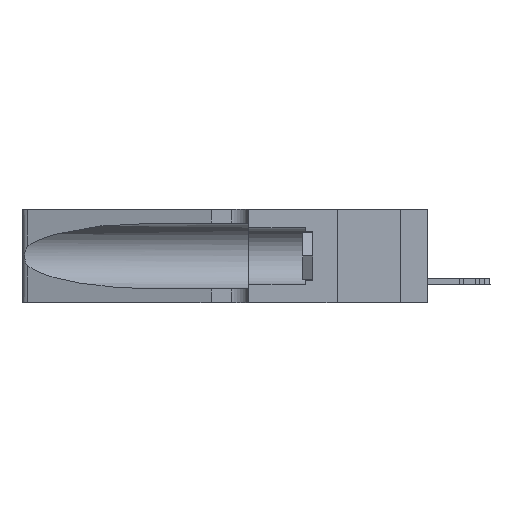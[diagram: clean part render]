
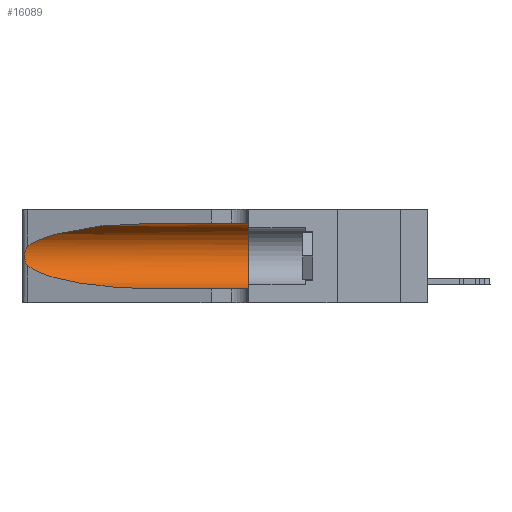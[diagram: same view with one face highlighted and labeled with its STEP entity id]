
A CAD part, left-side view. The second image highlights one B-rep face of the part: STEP entity #16089.
In plain terms, the highlighted cylindrical face has radius 3.308 mm (diameter 6.617 mm), a partial arc.
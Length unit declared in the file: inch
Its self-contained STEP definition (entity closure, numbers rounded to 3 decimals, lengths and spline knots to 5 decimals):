
#1194 = CARTESIAN_POINT ( 'NONE',  ( 0.26075, 1.23896, 0.178 ) ) ;
#1199 = EDGE_CURVE ( 'NONE', #40765, #4645, #34732, .T. ) ;
#1422 = CARTESIAN_POINT ( 'NONE',  ( 0.2373, 1.15595, 0.08982 ) ) ;
#1483 = VECTOR ( 'NONE', #41429, 39.37008 ) ;
#3904 =( BOUNDED_CURVE ( )  B_SPLINE_CURVE ( 3, ( #12185, #24140, #12664, #39968 ),
 .UNSPECIFIED., .F., .F. ) 
 B_SPLINE_CURVE_WITH_KNOTS ( ( 4, 4 ),
 ( 1.5708, 2.84003 ),
 .UNSPECIFIED. ) 
 CURVE ( )  GEOMETRIC_REPRESENTATION_ITEM ( )  RATIONAL_B_SPLINE_CURVE ( ( 1., 0.87, 0.87, 1. ) ) 
 REPRESENTATION_ITEM ( '' )  );
#4634 = CYLINDRICAL_SURFACE ( 'NONE', #38845, 0.13025 ) ;
#4645 = VERTEX_POINT ( 'NONE', #6978 ) ;
#5437 = CARTESIAN_POINT ( 'NONE',  ( 0.25789, 1.23486, 0.15765 ) ) ;
#6538 = EDGE_CURVE ( 'NONE', #39353, #4645, #30060, .T. ) ;
#6978 = CARTESIAN_POINT ( 'NONE',  ( 0.1305, 0.35, 0.05475 ) ) ;
#7087 = DIRECTION ( 'NONE',  ( 0., 0., 1. ) ) ;
#8058 = CARTESIAN_POINT ( 'NONE',  ( 0.1305, 0.72297, 0.31525 ) ) ;
#8326 =( BOUNDED_CURVE ( )  B_SPLINE_CURVE ( 3, ( #21541, #1422, #41560, #21363 ),
 .UNSPECIFIED., .F., .F. ) 
 B_SPLINE_CURVE_WITH_KNOTS ( ( 4, 4 ),
 ( 3.44316, 4.71239 ),
 .UNSPECIFIED. ) 
 CURVE ( )  GEOMETRIC_REPRESENTATION_ITEM ( )  RATIONAL_B_SPLINE_CURVE ( ( 1., 0.87, 0.87, 1. ) ) 
 REPRESENTATION_ITEM ( '' )  );
#8593 = CARTESIAN_POINT ( 'NONE',  ( 0.26018, 1.23835, 0.19895 ) ) ;
#9312 = CARTESIAN_POINT ( 'NONE',  ( 0.1305, 1.61858, 0.05475 ) ) ;
#10115 = CARTESIAN_POINT ( 'NONE',  ( 0.1305, 0.35, 0.185 ) ) ;
#11326 = ORIENTED_EDGE ( 'NONE', *, *, #1199, .F. ) ;
#11652 = DIRECTION ( 'NONE',  ( 0., 0., -1. ) ) ;
#12185 = CARTESIAN_POINT ( 'NONE',  ( 0.1305, 0.72297, 0.31525 ) ) ;
#12664 = CARTESIAN_POINT ( 'NONE',  ( 0.2373, 1.15595, 0.28018 ) ) ;
#15272 = ORIENTED_EDGE ( 'NONE', *, *, #6538, .T. ) ;
#16042 = CARTESIAN_POINT ( 'NONE',  ( 0.25854, 1.2359, 0.20912 ) ) ;
#16089 = ADVANCED_FACE ( 'NONE', ( #41214 ), #4634, .F. ) ;
#18287 = VECTOR ( 'NONE', #40070, 39.37008 ) ;
#19388 = ORIENTED_EDGE ( 'NONE', *, *, #27018, .T. ) ;
#21363 = CARTESIAN_POINT ( 'NONE',  ( 0.1305, 0.72297, 0.05475 ) ) ;
#21495 = DIRECTION ( 'NONE',  ( 0., 1., 0. ) ) ;
#21541 = CARTESIAN_POINT ( 'NONE',  ( 0.25487, 1.22718, 0.14631 ) ) ;
#22404 = VERTEX_POINT ( 'NONE', #8058 ) ;
#22653 = LINE ( 'NONE', #35394, #18287 ) ;
#22908 = CARTESIAN_POINT ( 'NONE',  ( 0.25487, 1.22718, 0.14631 ) ) ;
#23825 = CARTESIAN_POINT ( 'NONE',  ( 0.25555, 1.22994, 0.2215 ) ) ;
#24140 = CARTESIAN_POINT ( 'NONE',  ( 0.18966, 0.96281, 0.31525 ) ) ;
#24688 = EDGE_CURVE ( 'NONE', #22404, #36125, #3904, .T. ) ;
#24886 = EDGE_CURVE ( 'NONE', #22404, #40765, #22653, .T. ) ;
#27018 = EDGE_CURVE ( 'NONE', #36287, #39353, #8326, .T. ) ;
#28216 = CARTESIAN_POINT ( 'NONE',  ( 0.25487, 1.22718, 0.22369 ) ) ;
#28468 = CARTESIAN_POINT ( 'NONE',  ( 0.26075, 1.23896, 0.19203 ) ) ;
#28742 = CARTESIAN_POINT ( 'NONE',  ( 0.1305, 0.35, 0.31525 ) ) ;
#30060 = LINE ( 'NONE', #9312, #1483 ) ;
#31807 = CARTESIAN_POINT ( 'NONE',  ( 0.25487, 1.22718, 0.22369 ) ) ;
#32041 = EDGE_CURVE ( 'NONE', #36125, #36287, #50399, .T. ) ;
#34732 = CIRCLE ( 'NONE', #35881, 0.13025 ) ;
#35394 = CARTESIAN_POINT ( 'NONE',  ( 0.1305, 1.61858, 0.31525 ) ) ;
#35628 = ORIENTED_EDGE ( 'NONE', *, *, #24886, .F. ) ;
#35881 = AXIS2_PLACEMENT_3D ( 'NONE', #10115, #21495, #7087 ) ;
#36125 = VERTEX_POINT ( 'NONE', #31807 ) ;
#36287 = VERTEX_POINT ( 'NONE', #22908 ) ;
#36346 = CARTESIAN_POINT ( 'NONE',  ( 0.26017, 1.23833, 0.17102 ) ) ;
#36853 = CARTESIAN_POINT ( 'NONE',  ( 0.1305, 0.72297, 0.05475 ) ) ;
#37176 = ORIENTED_EDGE ( 'NONE', *, *, #24688, .T. ) ;
#38845 = AXIS2_PLACEMENT_3D ( 'NONE', #50130, #46670, #11652 ) ;
#39353 = VERTEX_POINT ( 'NONE', #36853 ) ;
#39968 = CARTESIAN_POINT ( 'NONE',  ( 0.25487, 1.22718, 0.22369 ) ) ;
#40070 = DIRECTION ( 'NONE',  ( 0., -1., 0. ) ) ;
#40263 = CARTESIAN_POINT ( 'NONE',  ( 0.25639, 1.23184, 0.21858 ) ) ;
#40425 = ORIENTED_EDGE ( 'NONE', *, *, #32041, .T. ) ;
#40765 = VERTEX_POINT ( 'NONE', #28742 ) ;
#41214 = FACE_OUTER_BOUND ( 'NONE', #43995, .T. ) ;
#41429 = DIRECTION ( 'NONE',  ( 0., -1., 0. ) ) ;
#41560 = CARTESIAN_POINT ( 'NONE',  ( 0.18966, 0.96281, 0.05475 ) ) ;
#43472 = CARTESIAN_POINT ( 'NONE',  ( 0.25787, 1.23484, 0.2124 ) ) ;
#43995 = EDGE_LOOP ( 'NONE', ( #37176, #40425, #19388, #15272, #11326, #35628 ) ) ;
#44213 = CARTESIAN_POINT ( 'NONE',  ( 0.25639, 1.23186, 0.15144 ) ) ;
#46670 = DIRECTION ( 'NONE',  ( 0., -1., 0. ) ) ;
#48694 = CARTESIAN_POINT ( 'NONE',  ( 0.25856, 1.23593, 0.16098 ) ) ;
#49439 = CARTESIAN_POINT ( 'NONE',  ( 0.25555, 1.22993, 0.14849 ) ) ;
#49635 = CARTESIAN_POINT ( 'NONE',  ( 0.25487, 1.22718, 0.14631 ) ) ;
#50130 = CARTESIAN_POINT ( 'NONE',  ( 0.1305, 1.61858, 0.185 ) ) ;
#50399 = B_SPLINE_CURVE_WITH_KNOTS ( 'NONE', 3,
 ( #28216, #23825, #40263, #43472, #16042, #8593, #28468, #1194, #36346, #48694, #5437, #44213, #49439, #49635 ),
 .UNSPECIFIED., .F., .F.,
 ( 4, 2, 2, 2, 2, 2, 4 ),
 ( 0., 0.00027, 0.00053, 0.00107, 0.0016, 0.00187, 0.00214 ),
 .UNSPECIFIED. ) ;
